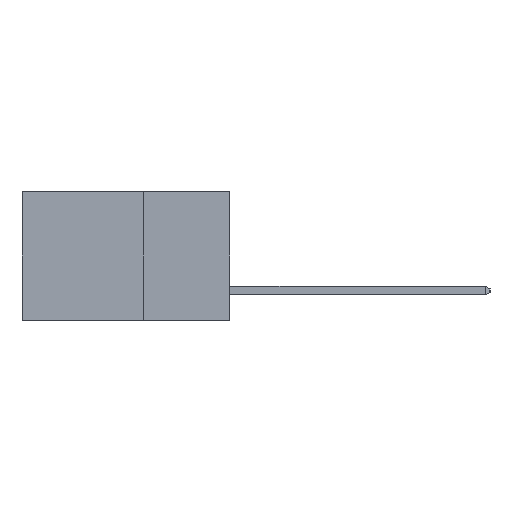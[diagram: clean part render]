
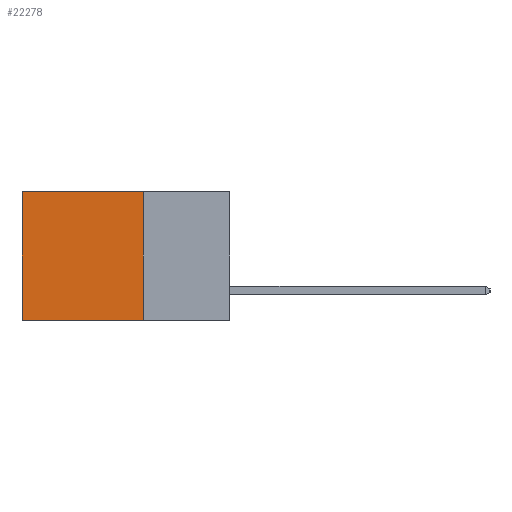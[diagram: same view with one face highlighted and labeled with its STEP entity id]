
A CAD part, left-side view. The second image highlights one B-rep face of the part: STEP entity #22278.
In plain terms, the highlighted planar face has unit normal (-1, 0, 0).
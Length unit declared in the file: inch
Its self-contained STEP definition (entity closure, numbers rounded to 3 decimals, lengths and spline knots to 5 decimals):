
#272 = CARTESIAN_POINT ( 'NONE',  ( 0.298, 0.6, 0. ) ) ;
#1069 = ORIENTED_EDGE ( 'NONE', *, *, #5834, .F. ) ;
#2006 = DIRECTION ( 'NONE',  ( 0., 0., -1. ) ) ;
#2217 = VERTEX_POINT ( 'NONE', #5848 ) ;
#2359 = LINE ( 'NONE', #272, #15084 ) ;
#3728 = ORIENTED_EDGE ( 'NONE', *, *, #6999, .T. ) ;
#4228 = EDGE_CURVE ( 'NONE', #7468, #14661, #6016, .T. ) ;
#4317 = VECTOR ( 'NONE', #16611, 39.37008 ) ;
#4366 = CARTESIAN_POINT ( 'NONE',  ( 0.298, 0.25, -0.37 ) ) ;
#5834 = EDGE_CURVE ( 'NONE', #17084, #7468, #13505, .T. ) ;
#5848 = CARTESIAN_POINT ( 'NONE',  ( 0.298, 0.6, 0. ) ) ;
#5914 = PLANE ( 'NONE',  #15382 ) ;
#5988 = DIRECTION ( 'NONE',  ( 1., 0., 0. ) ) ;
#6006 = VECTOR ( 'NONE', #14052, 39.37008 ) ;
#6016 = LINE ( 'NONE', #4366, #14646 ) ;
#6999 = EDGE_CURVE ( 'NONE', #2217, #14661, #2359, .T. ) ;
#7468 = VERTEX_POINT ( 'NONE', #18687 ) ;
#8712 = ORIENTED_EDGE ( 'NONE', *, *, #11974, .T. ) ;
#10597 = LINE ( 'NONE', #20934, #6006 ) ;
#11974 = EDGE_CURVE ( 'NONE', #17084, #2217, #10597, .T. ) ;
#12635 = FACE_OUTER_BOUND ( 'NONE', #18055, .T. ) ;
#12840 = CARTESIAN_POINT ( 'NONE',  ( 0.298, 0.25, 0. ) ) ;
#13505 = LINE ( 'NONE', #15484, #4317 ) ;
#14052 = DIRECTION ( 'NONE',  ( 0., 1., 0. ) ) ;
#14646 = VECTOR ( 'NONE', #21751, 39.37008 ) ;
#14661 = VERTEX_POINT ( 'NONE', #15366 ) ;
#15084 = VECTOR ( 'NONE', #2006, 39.37008 ) ;
#15205 = CARTESIAN_POINT ( 'NONE',  ( 0.298, 0.25, 0. ) ) ;
#15366 = CARTESIAN_POINT ( 'NONE',  ( 0.298, 0.6, -0.37 ) ) ;
#15382 = AXIS2_PLACEMENT_3D ( 'NONE', #12840, #5988, #18049 ) ;
#15484 = CARTESIAN_POINT ( 'NONE',  ( 0.298, 0.25, 0. ) ) ;
#16611 = DIRECTION ( 'NONE',  ( 0., 0., -1. ) ) ;
#17084 = VERTEX_POINT ( 'NONE', #15205 ) ;
#18049 = DIRECTION ( 'NONE',  ( 0., 0., -1. ) ) ;
#18055 = EDGE_LOOP ( 'NONE', ( #3728, #19518, #1069, #8712 ) ) ;
#18687 = CARTESIAN_POINT ( 'NONE',  ( 0.298, 0.25, -0.37 ) ) ;
#19518 = ORIENTED_EDGE ( 'NONE', *, *, #4228, .F. ) ;
#20934 = CARTESIAN_POINT ( 'NONE',  ( 0.298, 0.25, 0. ) ) ;
#21751 = DIRECTION ( 'NONE',  ( 0., 1., 0. ) ) ;
#22278 = ADVANCED_FACE ( 'NONE', ( #12635 ), #5914, .F. ) ;
